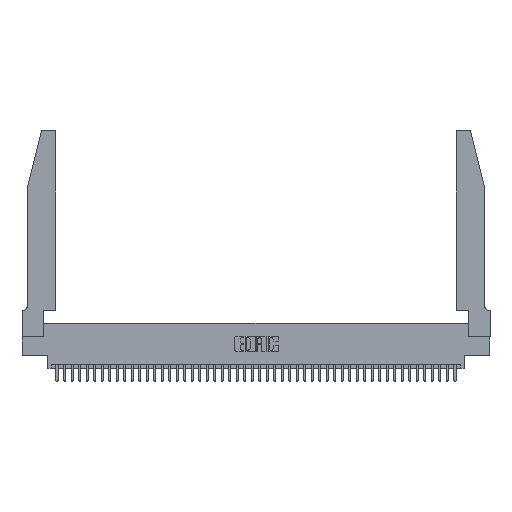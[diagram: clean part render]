
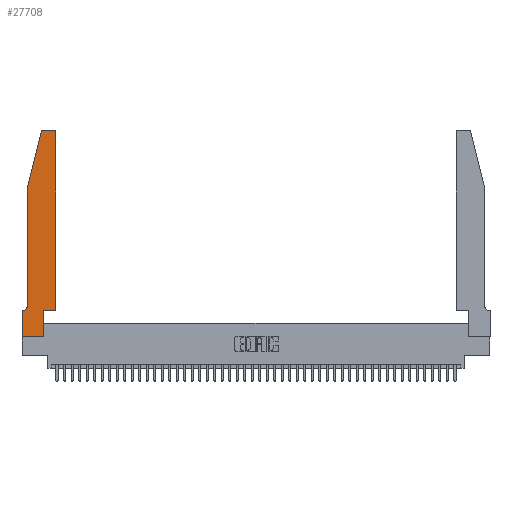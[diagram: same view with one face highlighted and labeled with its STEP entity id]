
A CAD part, top view. The second image highlights one B-rep face of the part: STEP entity #27708.
In plain terms, the highlighted planar face has unit normal (0, 0, 1).
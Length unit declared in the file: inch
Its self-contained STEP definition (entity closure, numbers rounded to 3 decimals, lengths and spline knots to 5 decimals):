
#136 = ORIENTED_EDGE ( 'NONE', *, *, #18813, .T. ) ;
#381 = EDGE_CURVE ( 'NONE', #10488, #31254, #21078, .T. ) ;
#1387 = CARTESIAN_POINT ( 'NONE',  ( 0.25487, 2.72718, 0.37 ) ) ;
#1392 = CARTESIAN_POINT ( 'NONE',  ( 0.0755, 0.42, 0.37 ) ) ;
#1539 = VECTOR ( 'NONE', #22653, 39.37008 ) ;
#1568 = CARTESIAN_POINT ( 'NONE',  ( 0., 0., 0.37 ) ) ;
#2970 = EDGE_LOOP ( 'NONE', ( #25168, #19866, #136, #20515, #42498, #7515, #16874, #25236, #28191, #23133, #41248, #37033 ) ) ;
#3208 = EDGE_CURVE ( 'NONE', #24349, #28793, #8005, .T. ) ;
#3730 = CIRCLE ( 'NONE', #12699, 0.03 ) ;
#3818 = AXIS2_PLACEMENT_3D ( 'NONE', #13232, #34144, #42142 ) ;
#4105 = CARTESIAN_POINT ( 'NONE',  ( 0.4505, 2.72, 0.37 ) ) ;
#4624 = LINE ( 'NONE', #27858, #37287 ) ;
#4676 = DIRECTION ( 'NONE',  ( 0., 1., 0. ) ) ;
#5521 = FACE_OUTER_BOUND ( 'NONE', #2970, .T. ) ;
#5612 = LINE ( 'NONE', #23080, #38248 ) ;
#5882 = DIRECTION ( 'NONE',  ( 0., 0., 1. ) ) ;
#6354 = CARTESIAN_POINT ( 'NONE',  ( 0.2605, 2.75, 0.37 ) ) ;
#6966 = VERTEX_POINT ( 'NONE', #34300 ) ;
#7515 = ORIENTED_EDGE ( 'NONE', *, *, #17139, .T. ) ;
#8005 = LINE ( 'NONE', #22360, #29015 ) ;
#8157 = LINE ( 'NONE', #43796, #24797 ) ;
#8759 = PLANE ( 'NONE',  #3818 ) ;
#9690 = EDGE_CURVE ( 'NONE', #14638, #24349, #8157, .T. ) ;
#9762 = DIRECTION ( 'NONE',  ( 0., -1., 0. ) ) ;
#10488 = VERTEX_POINT ( 'NONE', #1392 ) ;
#10604 = AXIS2_PLACEMENT_3D ( 'NONE', #40212, #19082, #29078 ) ;
#11019 = EDGE_CURVE ( 'NONE', #24253, #15159, #4624, .T. ) ;
#12687 = CARTESIAN_POINT ( 'NONE',  ( 0.284, 2.72, 0.37 ) ) ;
#12699 = AXIS2_PLACEMENT_3D ( 'NONE', #12687, #5882, #23850 ) ;
#13232 = CARTESIAN_POINT ( 'NONE',  ( 0., 0.35, 0.37 ) ) ;
#14401 = DIRECTION ( 'NONE',  ( -1., 0., 0. ) ) ;
#14638 = VERTEX_POINT ( 'NONE', #28123 ) ;
#15159 = VERTEX_POINT ( 'NONE', #41909 ) ;
#15259 = EDGE_CURVE ( 'NONE', #15159, #14638, #34758, .T. ) ;
#15465 = LINE ( 'NONE', #6354, #19349 ) ;
#16874 = ORIENTED_EDGE ( 'NONE', *, *, #11019, .T. ) ;
#17139 = EDGE_CURVE ( 'NONE', #31254, #24253, #5612, .T. ) ;
#17768 = CARTESIAN_POINT ( 'NONE',  ( 0.0055, 0.35, 0.37 ) ) ;
#17892 = VECTOR ( 'NONE', #21841, 39.37008 ) ;
#18004 = CARTESIAN_POINT ( 'NONE',  ( 0.0755, 2., 0.37 ) ) ;
#18385 = CARTESIAN_POINT ( 'NONE',  ( 0.0755, 2., 0.37 ) ) ;
#18610 = DIRECTION ( 'NONE',  ( -0.239, -0.971, 0. ) ) ;
#18813 = EDGE_CURVE ( 'NONE', #26270, #41430, #26456, .T. ) ;
#19082 = DIRECTION ( 'NONE',  ( 0., 0., -1. ) ) ;
#19349 = VECTOR ( 'NONE', #14401, 39.37008 ) ;
#19370 = CARTESIAN_POINT ( 'NONE',  ( 0.4505, 0.35, 0.37 ) ) ;
#19604 = DIRECTION ( 'NONE',  ( 1., 0., 0. ) ) ;
#19866 = ORIENTED_EDGE ( 'NONE', *, *, #39756, .T. ) ;
#20515 = ORIENTED_EDGE ( 'NONE', *, *, #42664, .T. ) ;
#21078 = CIRCLE ( 'NONE', #10604, 0.07 ) ;
#21531 = VECTOR ( 'NONE', #18610, 39.37008 ) ;
#21841 = DIRECTION ( 'NONE',  ( 0., -1., 0. ) ) ;
#22140 = CARTESIAN_POINT ( 'NONE',  ( 0., 0.35, 0.37 ) ) ;
#22360 = CARTESIAN_POINT ( 'NONE',  ( 0.4505, 0.35, 0.37 ) ) ;
#22653 = DIRECTION ( 'NONE',  ( 1., 0., 0. ) ) ;
#23080 = CARTESIAN_POINT ( 'NONE',  ( 0.0755, 0.35, 0.37 ) ) ;
#23133 = ORIENTED_EDGE ( 'NONE', *, *, #3208, .T. ) ;
#23850 = DIRECTION ( 'NONE',  ( 1., 0., 0. ) ) ;
#24253 = VERTEX_POINT ( 'NONE', #22140 ) ;
#24349 = VERTEX_POINT ( 'NONE', #34461 ) ;
#24797 = VECTOR ( 'NONE', #41032, 39.37008 ) ;
#25168 = ORIENTED_EDGE ( 'NONE', *, *, #27890, .T. ) ;
#25236 = ORIENTED_EDGE ( 'NONE', *, *, #15259, .T. ) ;
#26270 = VERTEX_POINT ( 'NONE', #1387 ) ;
#26456 = LINE ( 'NONE', #42854, #21531 ) ;
#26571 = VERTEX_POINT ( 'NONE', #4105 ) ;
#26757 = DIRECTION ( 'NONE',  ( -1., 0., 0. ) ) ;
#27708 = ADVANCED_FACE ( 'NONE', ( #5521 ), #8759, .T. ) ;
#27858 = CARTESIAN_POINT ( 'NONE',  ( 0., 0., 0.37 ) ) ;
#27890 = EDGE_CURVE ( 'NONE', #38305, #6966, #15465, .T. ) ;
#28123 = CARTESIAN_POINT ( 'NONE',  ( 0.2865, 0., 0.37 ) ) ;
#28191 = ORIENTED_EDGE ( 'NONE', *, *, #9690, .T. ) ;
#28459 = CIRCLE ( 'NONE', #43710, 0.03 ) ;
#28793 = VERTEX_POINT ( 'NONE', #19370 ) ;
#29015 = VECTOR ( 'NONE', #19604, 39.37008 ) ;
#29078 = DIRECTION ( 'NONE',  ( -1., 0., 0. ) ) ;
#30376 = LINE ( 'NONE', #43178, #45315 ) ;
#31254 = VERTEX_POINT ( 'NONE', #17768 ) ;
#32402 = DIRECTION ( 'NONE',  ( 1., 0., 0. ) ) ;
#33196 = EDGE_CURVE ( 'NONE', #28793, #26571, #30376, .T. ) ;
#34144 = DIRECTION ( 'NONE',  ( 0., 0., 1. ) ) ;
#34300 = CARTESIAN_POINT ( 'NONE',  ( 0.284, 2.75, 0.37 ) ) ;
#34461 = CARTESIAN_POINT ( 'NONE',  ( 0.2865, 0.35, 0.37 ) ) ;
#34758 = LINE ( 'NONE', #1568, #1539 ) ;
#35826 = DIRECTION ( 'NONE',  ( 0., 0., 1. ) ) ;
#37033 = ORIENTED_EDGE ( 'NONE', *, *, #43214, .T. ) ;
#37287 = VECTOR ( 'NONE', #9762, 39.37008 ) ;
#38248 = VECTOR ( 'NONE', #26757, 39.37008 ) ;
#38305 = VERTEX_POINT ( 'NONE', #41085 ) ;
#39230 = CARTESIAN_POINT ( 'NONE',  ( 0.4205, 2.72, 0.37 ) ) ;
#39416 = LINE ( 'NONE', #18004, #17892 ) ;
#39756 = EDGE_CURVE ( 'NONE', #6966, #26270, #3730, .T. ) ;
#40212 = CARTESIAN_POINT ( 'NONE',  ( 0.0055, 0.42, 0.37 ) ) ;
#41032 = DIRECTION ( 'NONE',  ( 0., 1., 0. ) ) ;
#41085 = CARTESIAN_POINT ( 'NONE',  ( 0.4205, 2.75, 0.37 ) ) ;
#41248 = ORIENTED_EDGE ( 'NONE', *, *, #33196, .T. ) ;
#41430 = VERTEX_POINT ( 'NONE', #18385 ) ;
#41909 = CARTESIAN_POINT ( 'NONE',  ( 0., 0., 0.37 ) ) ;
#42142 = DIRECTION ( 'NONE',  ( 1., 0., 0. ) ) ;
#42498 = ORIENTED_EDGE ( 'NONE', *, *, #381, .T. ) ;
#42664 = EDGE_CURVE ( 'NONE', #41430, #10488, #39416, .T. ) ;
#42854 = CARTESIAN_POINT ( 'NONE',  ( 0.0755, 2., 0.37 ) ) ;
#43178 = CARTESIAN_POINT ( 'NONE',  ( 0.4505, 0.35, 0.37 ) ) ;
#43214 = EDGE_CURVE ( 'NONE', #26571, #38305, #28459, .T. ) ;
#43710 = AXIS2_PLACEMENT_3D ( 'NONE', #39230, #35826, #32402 ) ;
#43796 = CARTESIAN_POINT ( 'NONE',  ( 0.2865, 0.35, 0.37 ) ) ;
#45315 = VECTOR ( 'NONE', #4676, 39.37008 ) ;
